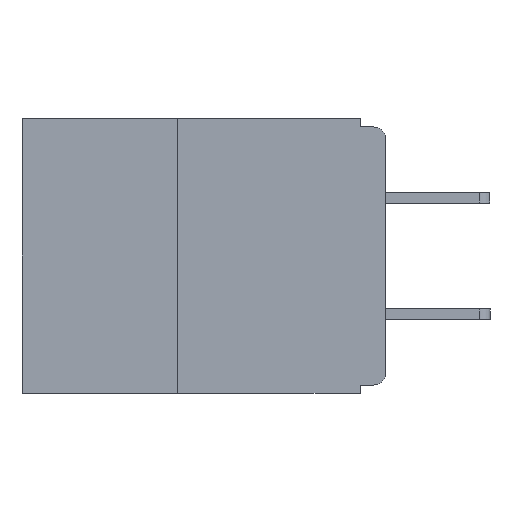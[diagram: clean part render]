
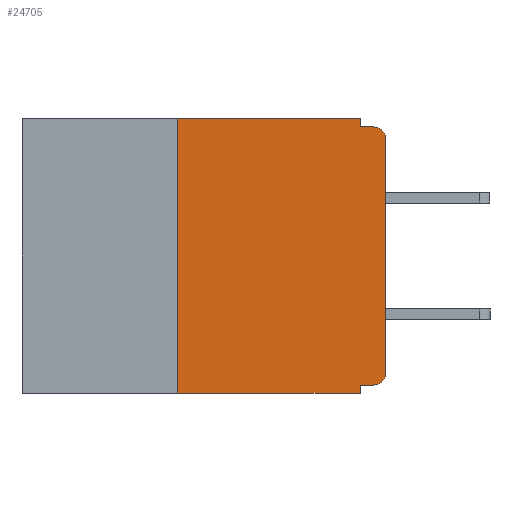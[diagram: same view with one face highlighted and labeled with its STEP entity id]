
A CAD part, left-side view. The second image highlights one B-rep face of the part: STEP entity #24705.
In plain terms, the highlighted planar face has unit normal (-1, 0, 0).
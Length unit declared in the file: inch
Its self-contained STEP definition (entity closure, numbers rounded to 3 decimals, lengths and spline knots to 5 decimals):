
#88 = DIRECTION ( 'NONE',  ( 0., 0., -1. ) ) ;
#371 = VECTOR ( 'NONE', #4998, 39.37008 ) ;
#502 = VECTOR ( 'NONE', #3339, 39.37008 ) ;
#602 = VERTEX_POINT ( 'NONE', #12048 ) ;
#639 = PLANE ( 'NONE',  #25618 ) ;
#740 = ORIENTED_EDGE ( 'NONE', *, *, #10687, .T. ) ;
#1198 = LINE ( 'NONE', #15474, #502 ) ;
#1206 = ORIENTED_EDGE ( 'NONE', *, *, #22531, .F. ) ;
#1381 = CARTESIAN_POINT ( 'NONE',  ( 0., 0., -0.025 ) ) ;
#1637 = EDGE_CURVE ( 'NONE', #5814, #3490, #12680, .T. ) ;
#2128 = CARTESIAN_POINT ( 'NONE',  ( 0., 0.015, -0.01 ) ) ;
#2252 = LINE ( 'NONE', #11102, #17886 ) ;
#2365 = EDGE_CURVE ( 'NONE', #5796, #5405, #12967, .T. ) ;
#2551 = ORIENTED_EDGE ( 'NONE', *, *, #25286, .F. ) ;
#2707 = AXIS2_PLACEMENT_3D ( 'NONE', #21005, #20858, #20825 ) ;
#2825 = VERTEX_POINT ( 'NONE', #14294 ) ;
#2883 = CARTESIAN_POINT ( 'NONE',  ( 0., 0., -0.01 ) ) ;
#3075 = EDGE_CURVE ( 'NONE', #4051, #2825, #2252, .T. ) ;
#3339 = DIRECTION ( 'NONE',  ( 0., 0., -1. ) ) ;
#3366 = ORIENTED_EDGE ( 'NONE', *, *, #7515, .T. ) ;
#3490 = VERTEX_POINT ( 'NONE', #5429 ) ;
#3986 = ORIENTED_EDGE ( 'NONE', *, *, #1637, .F. ) ;
#4051 = VERTEX_POINT ( 'NONE', #26056 ) ;
#4792 = CARTESIAN_POINT ( 'NONE',  ( 0., 0., -0.305 ) ) ;
#4998 = DIRECTION ( 'NONE',  ( 0., -1., 0. ) ) ;
#5153 = VECTOR ( 'NONE', #6005, 39.37008 ) ;
#5349 = AXIS2_PLACEMENT_3D ( 'NONE', #24441, #12600, #88 ) ;
#5405 = VERTEX_POINT ( 'NONE', #4792 ) ;
#5429 = CARTESIAN_POINT ( 'NONE',  ( 0., 0.25, 0. ) ) ;
#5796 = VERTEX_POINT ( 'NONE', #13087 ) ;
#5814 = VERTEX_POINT ( 'NONE', #7039 ) ;
#6005 = DIRECTION ( 'NONE',  ( 0., -1., 0. ) ) ;
#6440 = VECTOR ( 'NONE', #10280, 39.37008 ) ;
#6562 = VECTOR ( 'NONE', #6597, 39.37008 ) ;
#6581 = VERTEX_POINT ( 'NONE', #1381 ) ;
#6597 = DIRECTION ( 'NONE',  ( 0., 0., 1. ) ) ;
#7005 = ORIENTED_EDGE ( 'NONE', *, *, #2365, .T. ) ;
#7039 = CARTESIAN_POINT ( 'NONE',  ( 0., 0.25, -0.33 ) ) ;
#7290 = VECTOR ( 'NONE', #18521, 39.37008 ) ;
#7515 = EDGE_CURVE ( 'NONE', #5405, #6581, #22544, .T. ) ;
#7655 = CARTESIAN_POINT ( 'NONE',  ( 0., 0.031, -0.33 ) ) ;
#8683 = VERTEX_POINT ( 'NONE', #7655 ) ;
#10280 = DIRECTION ( 'NONE',  ( 0., 1., 0. ) ) ;
#10687 = EDGE_CURVE ( 'NONE', #6581, #16516, #23192, .T. ) ;
#10819 = VECTOR ( 'NONE', #15986, 39.37008 ) ;
#10917 = DIRECTION ( 'NONE',  ( 0., 0., -1. ) ) ;
#11102 = CARTESIAN_POINT ( 'NONE',  ( 0., 0.031, 0. ) ) ;
#11209 = EDGE_LOOP ( 'NONE', ( #3366, #740, #2551, #13163, #22224, #3986, #21424, #1206, #21991, #7005 ) ) ;
#11258 = LINE ( 'NONE', #12080, #5153 ) ;
#11500 = LINE ( 'NONE', #2883, #371 ) ;
#11872 = LINE ( 'NONE', #20238, #6440 ) ;
#12048 = CARTESIAN_POINT ( 'NONE',  ( 0., 0.031, -0.32 ) ) ;
#12080 = CARTESIAN_POINT ( 'NONE',  ( 0., 0.437, -0.33 ) ) ;
#12600 = DIRECTION ( 'NONE',  ( -1., 0., 0. ) ) ;
#12680 = LINE ( 'NONE', #18925, #7290 ) ;
#12967 = CIRCLE ( 'NONE', #2707, 0.015 ) ;
#13087 = CARTESIAN_POINT ( 'NONE',  ( 0., 0.015, -0.32 ) ) ;
#13163 = ORIENTED_EDGE ( 'NONE', *, *, #3075, .F. ) ;
#13181 = DIRECTION ( 'NONE',  ( 0., 0., -1. ) ) ;
#13448 = EDGE_CURVE ( 'NONE', #5796, #602, #11872, .T. ) ;
#14294 = CARTESIAN_POINT ( 'NONE',  ( 0., 0.031, -0.01 ) ) ;
#15224 = EDGE_CURVE ( 'NONE', #3490, #4051, #25950, .T. ) ;
#15474 = CARTESIAN_POINT ( 'NONE',  ( 0., 0.031, -0.33 ) ) ;
#15986 = DIRECTION ( 'NONE',  ( 0., -1., 0. ) ) ;
#16516 = VERTEX_POINT ( 'NONE', #2128 ) ;
#17886 = VECTOR ( 'NONE', #10917, 39.37008 ) ;
#18521 = DIRECTION ( 'NONE',  ( 0., 0., 1. ) ) ;
#18925 = CARTESIAN_POINT ( 'NONE',  ( 0., 0.25, -0.33 ) ) ;
#19061 = CARTESIAN_POINT ( 'NONE',  ( 0., 0.437, 0. ) ) ;
#20238 = CARTESIAN_POINT ( 'NONE',  ( 0., 0., -0.32 ) ) ;
#20825 = DIRECTION ( 'NONE',  ( 0., 0., -1. ) ) ;
#20858 = DIRECTION ( 'NONE',  ( -1., 0., 0. ) ) ;
#21005 = CARTESIAN_POINT ( 'NONE',  ( 0., 0.015, -0.305 ) ) ;
#21171 = FACE_OUTER_BOUND ( 'NONE', #11209, .T. ) ;
#21424 = ORIENTED_EDGE ( 'NONE', *, *, #23851, .T. ) ;
#21991 = ORIENTED_EDGE ( 'NONE', *, *, #13448, .F. ) ;
#22224 = ORIENTED_EDGE ( 'NONE', *, *, #15224, .F. ) ;
#22531 = EDGE_CURVE ( 'NONE', #602, #8683, #1198, .T. ) ;
#22544 = LINE ( 'NONE', #22624, #6562 ) ;
#22624 = CARTESIAN_POINT ( 'NONE',  ( 0., 0., 0. ) ) ;
#23192 = CIRCLE ( 'NONE', #5349, 0.015 ) ;
#23851 = EDGE_CURVE ( 'NONE', #5814, #8683, #11258, .T. ) ;
#24441 = CARTESIAN_POINT ( 'NONE',  ( 0., 0.015, -0.025 ) ) ;
#24705 = ADVANCED_FACE ( 'NONE', ( #21171 ), #639, .F. ) ;
#24971 = DIRECTION ( 'NONE',  ( 1., 0., 0. ) ) ;
#25286 = EDGE_CURVE ( 'NONE', #2825, #16516, #11500, .T. ) ;
#25618 = AXIS2_PLACEMENT_3D ( 'NONE', #19061, #24971, #13181 ) ;
#25731 = CARTESIAN_POINT ( 'NONE',  ( 0., 0.437, 0. ) ) ;
#25950 = LINE ( 'NONE', #25731, #10819 ) ;
#26056 = CARTESIAN_POINT ( 'NONE',  ( 0., 0.031, 0. ) ) ;
